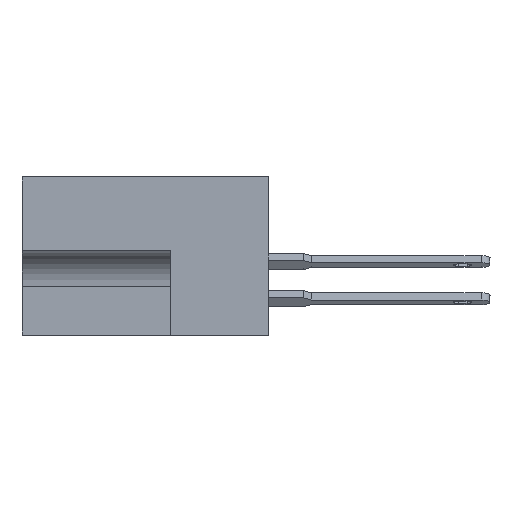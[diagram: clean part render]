
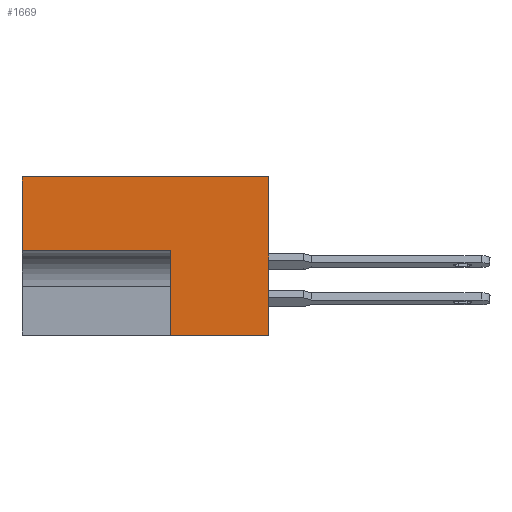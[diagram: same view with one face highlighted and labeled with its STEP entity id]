
A CAD part, left-side view. The second image highlights one B-rep face of the part: STEP entity #1669.
In plain terms, the highlighted planar face has unit normal (-1, 0, 0).
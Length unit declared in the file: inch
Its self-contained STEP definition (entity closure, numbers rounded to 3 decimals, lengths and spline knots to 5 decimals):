
#951 = DIRECTION ( 'NONE',  ( 1., 0., 0. ) ) ;
#1402 = VERTEX_POINT ( 'NONE', #10859 ) ;
#1408 = ORIENTED_EDGE ( 'NONE', *, *, #17683, .T. ) ;
#1501 = CARTESIAN_POINT ( 'NONE',  ( 0., 0.828, -0.248 ) ) ;
#1580 = AXIS2_PLACEMENT_3D ( 'NONE', #11789, #951, #18892 ) ;
#1669 = ADVANCED_FACE ( 'NONE', ( #23530 ), #9901, .F. ) ;
#1983 = LINE ( 'NONE', #2045, #14201 ) ;
#2045 = CARTESIAN_POINT ( 'NONE',  ( 0., 0.328, -0.248 ) ) ;
#2777 = ORIENTED_EDGE ( 'NONE', *, *, #4762, .F. ) ;
#2945 = EDGE_CURVE ( 'NONE', #13794, #1402, #18327, .T. ) ;
#4465 = VECTOR ( 'NONE', #7121, 39.37008 ) ;
#4762 = EDGE_CURVE ( 'NONE', #12765, #13794, #16158, .T. ) ;
#5127 = CARTESIAN_POINT ( 'NONE',  ( 0., 0.328, -0.531 ) ) ;
#5325 = VECTOR ( 'NONE', #16820, 39.37008 ) ;
#5518 = EDGE_LOOP ( 'NONE', ( #2777, #19450, #14335, #17533, #1408, #7928 ) ) ;
#5891 = VERTEX_POINT ( 'NONE', #12046 ) ;
#6165 = VERTEX_POINT ( 'NONE', #7802 ) ;
#6717 = VECTOR ( 'NONE', #9812, 39.37008 ) ;
#7067 = CARTESIAN_POINT ( 'NONE',  ( 0., 0.328, -0.248 ) ) ;
#7121 = DIRECTION ( 'NONE',  ( 0., 0., 1. ) ) ;
#7802 = CARTESIAN_POINT ( 'NONE',  ( 0., 0., -0.531 ) ) ;
#7822 = CARTESIAN_POINT ( 'NONE',  ( 0., 0.453, 0. ) ) ;
#7928 = ORIENTED_EDGE ( 'NONE', *, *, #2945, .F. ) ;
#8763 = CARTESIAN_POINT ( 'NONE',  ( 0., 0.828, 0. ) ) ;
#9436 = CARTESIAN_POINT ( 'NONE',  ( 0., 0., 0. ) ) ;
#9511 = DIRECTION ( 'NONE',  ( 0., -1., 0. ) ) ;
#9812 = DIRECTION ( 'NONE',  ( 0., -1., 0. ) ) ;
#9901 = PLANE ( 'NONE',  #1580 ) ;
#10162 = EDGE_CURVE ( 'NONE', #12319, #12765, #1983, .T. ) ;
#10170 = LINE ( 'NONE', #9436, #5325 ) ;
#10859 = CARTESIAN_POINT ( 'NONE',  ( 0., 0., 0. ) ) ;
#11789 = CARTESIAN_POINT ( 'NONE',  ( 0., 0.453, 0. ) ) ;
#12046 = CARTESIAN_POINT ( 'NONE',  ( 0., 0.328, -0.531 ) ) ;
#12319 = VERTEX_POINT ( 'NONE', #7067 ) ;
#12765 = VERTEX_POINT ( 'NONE', #1501 ) ;
#13252 = LINE ( 'NONE', #15244, #6717 ) ;
#13794 = VERTEX_POINT ( 'NONE', #8763 ) ;
#14201 = VECTOR ( 'NONE', #22127, 39.37008 ) ;
#14335 = ORIENTED_EDGE ( 'NONE', *, *, #17491, .F. ) ;
#15244 = CARTESIAN_POINT ( 'NONE',  ( 0., 0.453, -0.531 ) ) ;
#15686 = DIRECTION ( 'NONE',  ( 0., 0., 1. ) ) ;
#16158 = LINE ( 'NONE', #22756, #23544 ) ;
#16820 = DIRECTION ( 'NONE',  ( 0., 0., 1. ) ) ;
#17491 = EDGE_CURVE ( 'NONE', #5891, #12319, #20697, .T. ) ;
#17533 = ORIENTED_EDGE ( 'NONE', *, *, #17873, .T. ) ;
#17683 = EDGE_CURVE ( 'NONE', #6165, #1402, #10170, .T. ) ;
#17873 = EDGE_CURVE ( 'NONE', #5891, #6165, #13252, .T. ) ;
#18327 = LINE ( 'NONE', #7822, #22008 ) ;
#18892 = DIRECTION ( 'NONE',  ( 0., 0., -1. ) ) ;
#19450 = ORIENTED_EDGE ( 'NONE', *, *, #10162, .F. ) ;
#20697 = LINE ( 'NONE', #5127, #4465 ) ;
#22008 = VECTOR ( 'NONE', #9511, 39.37008 ) ;
#22127 = DIRECTION ( 'NONE',  ( 0., 1., 0. ) ) ;
#22756 = CARTESIAN_POINT ( 'NONE',  ( 0., 0.828, 0. ) ) ;
#23530 = FACE_OUTER_BOUND ( 'NONE', #5518, .T. ) ;
#23544 = VECTOR ( 'NONE', #15686, 39.37008 ) ;
